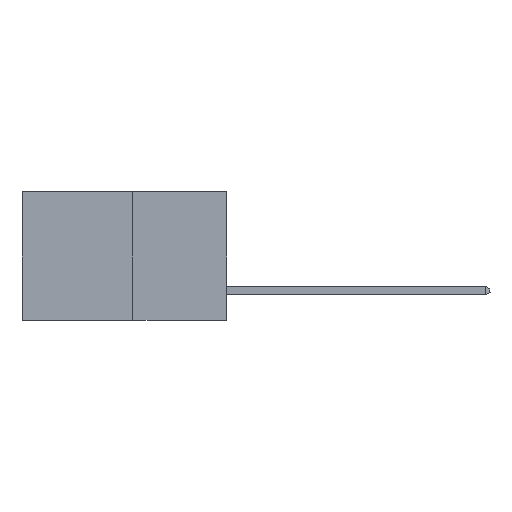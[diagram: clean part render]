
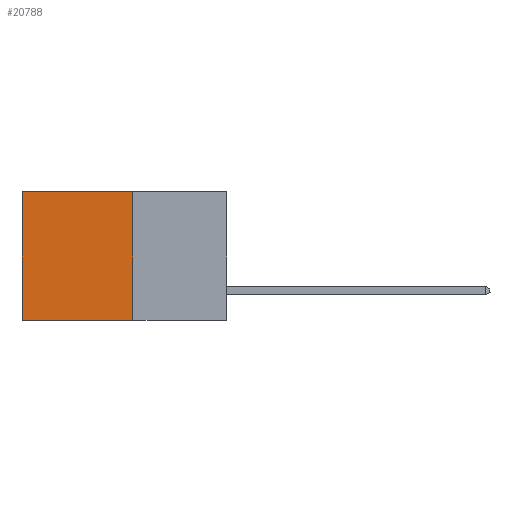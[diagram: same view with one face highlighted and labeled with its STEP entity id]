
A CAD part, left-side view. The second image highlights one B-rep face of the part: STEP entity #20788.
In plain terms, the highlighted planar face has unit normal (-1, 0, 0).
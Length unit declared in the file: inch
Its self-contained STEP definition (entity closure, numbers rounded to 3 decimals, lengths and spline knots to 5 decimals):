
#1273 = EDGE_CURVE ( 'NONE', #15932, #16098, #9897, .T. ) ;
#2047 = VECTOR ( 'NONE', #22171, 39.37008 ) ;
#3080 = LINE ( 'NONE', #3369, #8606 ) ;
#3369 = CARTESIAN_POINT ( 'NONE',  ( 0.277, 0.27, -0.37 ) ) ;
#4741 = AXIS2_PLACEMENT_3D ( 'NONE', #7522, #19875, #7616 ) ;
#4904 = DIRECTION ( 'NONE',  ( 0., 0., -1. ) ) ;
#6227 = DIRECTION ( 'NONE',  ( 0., 1., 0. ) ) ;
#6328 = CARTESIAN_POINT ( 'NONE',  ( 0.277, 0.27, 0. ) ) ;
#7522 = CARTESIAN_POINT ( 'NONE',  ( 0.277, 0.27, -0.37 ) ) ;
#7616 = DIRECTION ( 'NONE',  ( 0., 0., -1. ) ) ;
#7980 = CARTESIAN_POINT ( 'NONE',  ( 0.277, 0.27, -0.37 ) ) ;
#8606 = VECTOR ( 'NONE', #17813, 39.37008 ) ;
#9500 = CARTESIAN_POINT ( 'NONE',  ( 0.277, 0.59, 0. ) ) ;
#9897 = LINE ( 'NONE', #6328, #14753 ) ;
#12451 = LINE ( 'NONE', #7980, #2047 ) ;
#13650 = EDGE_CURVE ( 'NONE', #16098, #21237, #25297, .T. ) ;
#14753 = VECTOR ( 'NONE', #6227, 39.37008 ) ;
#15808 = PLANE ( 'NONE',  #4741 ) ;
#15932 = VERTEX_POINT ( 'NONE', #25085 ) ;
#16098 = VERTEX_POINT ( 'NONE', #9500 ) ;
#16143 = EDGE_CURVE ( 'NONE', #21958, #21237, #12451, .T. ) ;
#17813 = DIRECTION ( 'NONE',  ( 0., 0., -1. ) ) ;
#17999 = EDGE_LOOP ( 'NONE', ( #20248, #21696, #18515, #24266 ) ) ;
#18515 = ORIENTED_EDGE ( 'NONE', *, *, #23921, .F. ) ;
#19875 = DIRECTION ( 'NONE',  ( 1., 0., 0. ) ) ;
#20248 = ORIENTED_EDGE ( 'NONE', *, *, #13650, .T. ) ;
#20788 = ADVANCED_FACE ( 'NONE', ( #26069 ), #15808, .F. ) ;
#21231 = CARTESIAN_POINT ( 'NONE',  ( 0.277, 0.59, -0.37 ) ) ;
#21237 = VERTEX_POINT ( 'NONE', #21231 ) ;
#21282 = CARTESIAN_POINT ( 'NONE',  ( 0.277, 0.59, -0.37 ) ) ;
#21469 = CARTESIAN_POINT ( 'NONE',  ( 0.277, 0.27, -0.37 ) ) ;
#21696 = ORIENTED_EDGE ( 'NONE', *, *, #16143, .F. ) ;
#21958 = VERTEX_POINT ( 'NONE', #21469 ) ;
#22171 = DIRECTION ( 'NONE',  ( 0., 1., 0. ) ) ;
#23921 = EDGE_CURVE ( 'NONE', #15932, #21958, #3080, .T. ) ;
#24266 = ORIENTED_EDGE ( 'NONE', *, *, #1273, .T. ) ;
#25085 = CARTESIAN_POINT ( 'NONE',  ( 0.277, 0.27, 0. ) ) ;
#25297 = LINE ( 'NONE', #21282, #25891 ) ;
#25891 = VECTOR ( 'NONE', #4904, 39.37008 ) ;
#26069 = FACE_OUTER_BOUND ( 'NONE', #17999, .T. ) ;
